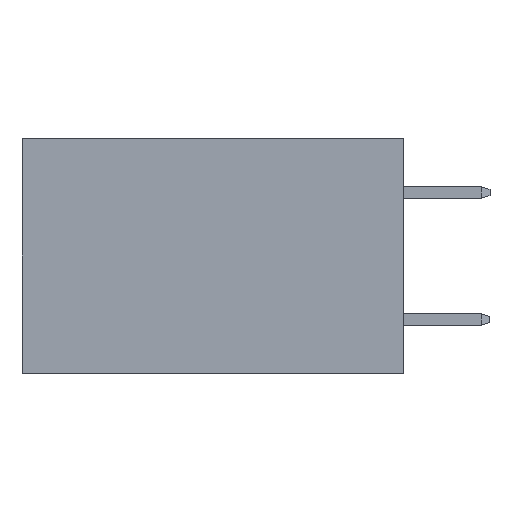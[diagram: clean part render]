
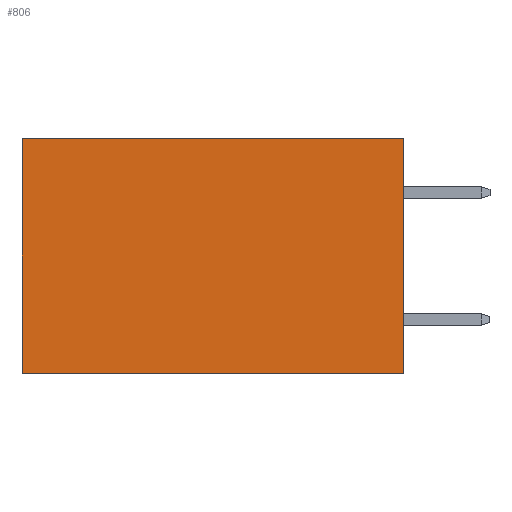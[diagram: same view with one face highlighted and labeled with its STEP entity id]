
A CAD part, left-side view. The second image highlights one B-rep face of the part: STEP entity #806.
In plain terms, the highlighted planar face has unit normal (-1, 0, 0).
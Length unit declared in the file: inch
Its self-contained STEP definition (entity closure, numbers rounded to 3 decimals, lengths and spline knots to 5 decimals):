
#57 = VECTOR ( 'NONE', #7922, 39.37008 ) ;
#406 = LINE ( 'NONE', #3665, #57 ) ;
#454 = DIRECTION ( 'NONE',  ( 0., 0., -1. ) ) ;
#494 = VERTEX_POINT ( 'NONE', #8803 ) ;
#806 = ADVANCED_FACE ( 'NONE', ( #953 ), #4124, .F. ) ;
#953 = FACE_OUTER_BOUND ( 'NONE', #6117, .T. ) ;
#1851 = EDGE_CURVE ( 'NONE', #7871, #6367, #2872, .T. ) ;
#2089 = VERTEX_POINT ( 'NONE', #8596 ) ;
#2102 = DIRECTION ( 'NONE',  ( 0., 1., 0. ) ) ;
#2296 = VECTOR ( 'NONE', #454, 39.37008 ) ;
#2355 = DIRECTION ( 'NONE',  ( 1., 0., 0. ) ) ;
#2627 = DIRECTION ( 'NONE',  ( 0., 0., -1. ) ) ;
#2872 = LINE ( 'NONE', #5336, #6603 ) ;
#3219 = EDGE_CURVE ( 'NONE', #494, #7871, #4523, .T. ) ;
#3320 = DIRECTION ( 'NONE',  ( 0., 0., -1. ) ) ;
#3439 = ORIENTED_EDGE ( 'NONE', *, *, #1851, .F. ) ;
#3665 = CARTESIAN_POINT ( 'NONE',  ( 0.2875, 0., 0. ) ) ;
#4124 = PLANE ( 'NONE',  #4674 ) ;
#4523 = LINE ( 'NONE', #7866, #2296 ) ;
#4674 = AXIS2_PLACEMENT_3D ( 'NONE', #6530, #2355, #3320 ) ;
#5336 = CARTESIAN_POINT ( 'NONE',  ( 0.2875, 0., -0.37 ) ) ;
#5701 = ORIENTED_EDGE ( 'NONE', *, *, #8440, .T. ) ;
#6016 = EDGE_CURVE ( 'NONE', #2089, #6367, #7618, .T. ) ;
#6117 = EDGE_LOOP ( 'NONE', ( #7744, #3439, #7269, #5701 ) ) ;
#6122 = VECTOR ( 'NONE', #2627, 39.37008 ) ;
#6367 = VERTEX_POINT ( 'NONE', #7387 ) ;
#6530 = CARTESIAN_POINT ( 'NONE',  ( 0.2875, 0., 0. ) ) ;
#6603 = VECTOR ( 'NONE', #2102, 39.37008 ) ;
#7269 = ORIENTED_EDGE ( 'NONE', *, *, #3219, .F. ) ;
#7355 = CARTESIAN_POINT ( 'NONE',  ( 0.2875, 0.6, 0. ) ) ;
#7387 = CARTESIAN_POINT ( 'NONE',  ( 0.2875, 0.6, -0.37 ) ) ;
#7566 = CARTESIAN_POINT ( 'NONE',  ( 0.2875, 0., -0.37 ) ) ;
#7618 = LINE ( 'NONE', #7355, #6122 ) ;
#7744 = ORIENTED_EDGE ( 'NONE', *, *, #6016, .T. ) ;
#7866 = CARTESIAN_POINT ( 'NONE',  ( 0.2875, 0., 0. ) ) ;
#7871 = VERTEX_POINT ( 'NONE', #7566 ) ;
#7922 = DIRECTION ( 'NONE',  ( 0., 1., 0. ) ) ;
#8440 = EDGE_CURVE ( 'NONE', #494, #2089, #406, .T. ) ;
#8596 = CARTESIAN_POINT ( 'NONE',  ( 0.2875, 0.6, 0. ) ) ;
#8803 = CARTESIAN_POINT ( 'NONE',  ( 0.2875, 0., 0. ) ) ;
